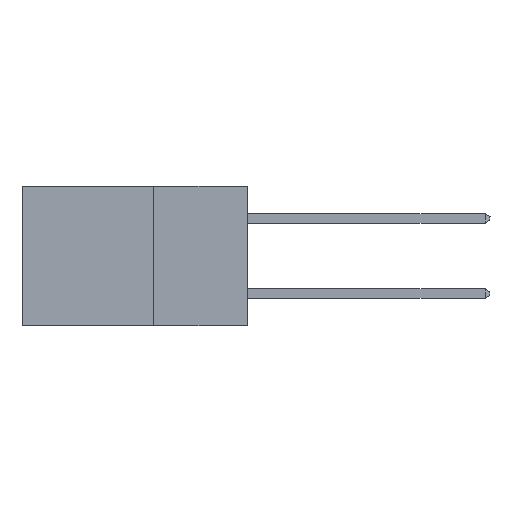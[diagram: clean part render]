
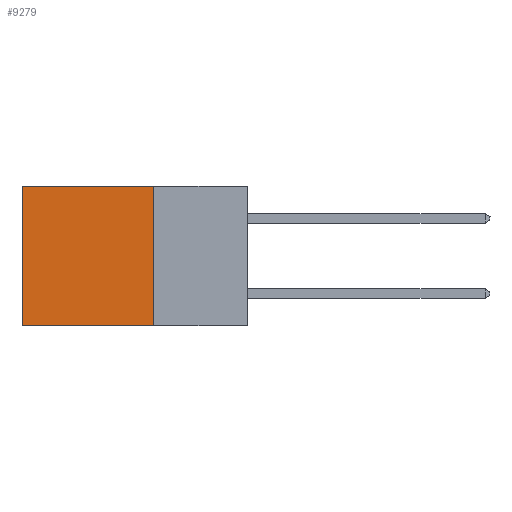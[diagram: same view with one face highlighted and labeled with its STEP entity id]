
A CAD part, left-side view. The second image highlights one B-rep face of the part: STEP entity #9279.
In plain terms, the highlighted planar face has unit normal (-1, 0, 0).
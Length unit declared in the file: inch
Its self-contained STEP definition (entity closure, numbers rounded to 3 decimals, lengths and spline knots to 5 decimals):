
#1099 = CARTESIAN_POINT ( 'NONE',  ( 0.2615, 0.6, -0.37 ) ) ;
#2013 = DIRECTION ( 'NONE',  ( 0., 1., 0. ) ) ;
#2723 = VECTOR ( 'NONE', #13078, 39.37008 ) ;
#2964 = VERTEX_POINT ( 'NONE', #15084 ) ;
#3114 = CARTESIAN_POINT ( 'NONE',  ( 0.2615, 0.25, -0.37 ) ) ;
#3133 = DIRECTION ( 'NONE',  ( 0., 0., -1. ) ) ;
#3724 = CARTESIAN_POINT ( 'NONE',  ( 0.2615, 0.6, 0. ) ) ;
#4052 = CARTESIAN_POINT ( 'NONE',  ( 0.2615, 0.25, -0.37 ) ) ;
#4297 = CARTESIAN_POINT ( 'NONE',  ( 0.2615, 0.6, -0.37 ) ) ;
#4444 = PLANE ( 'NONE',  #4728 ) ;
#4728 = AXIS2_PLACEMENT_3D ( 'NONE', #8635, #11301, #9491 ) ;
#5065 = ORIENTED_EDGE ( 'NONE', *, *, #6851, .T. ) ;
#5196 = EDGE_LOOP ( 'NONE', ( #5065, #15899, #11565, #14851 ) ) ;
#5509 = VECTOR ( 'NONE', #2013, 39.37008 ) ;
#6264 = EDGE_CURVE ( 'NONE', #2964, #8050, #11392, .T. ) ;
#6851 = EDGE_CURVE ( 'NONE', #14279, #11675, #14535, .T. ) ;
#7336 = EDGE_CURVE ( 'NONE', #2964, #14279, #8309, .T. ) ;
#7638 = CARTESIAN_POINT ( 'NONE',  ( 0.2615, 0.25, -0.37 ) ) ;
#8050 = VERTEX_POINT ( 'NONE', #4052 ) ;
#8309 = LINE ( 'NONE', #13406, #5509 ) ;
#8635 = CARTESIAN_POINT ( 'NONE',  ( 0.2615, 0.25, -0.37 ) ) ;
#9279 = ADVANCED_FACE ( 'NONE', ( #16297 ), #4444, .F. ) ;
#9491 = DIRECTION ( 'NONE',  ( 0., 0., -1. ) ) ;
#9801 = EDGE_CURVE ( 'NONE', #8050, #11675, #14704, .T. ) ;
#11045 = VECTOR ( 'NONE', #11546, 39.37008 ) ;
#11301 = DIRECTION ( 'NONE',  ( 1., 0., 0. ) ) ;
#11392 = LINE ( 'NONE', #7638, #11045 ) ;
#11546 = DIRECTION ( 'NONE',  ( 0., 0., -1. ) ) ;
#11565 = ORIENTED_EDGE ( 'NONE', *, *, #6264, .F. ) ;
#11675 = VERTEX_POINT ( 'NONE', #1099 ) ;
#13078 = DIRECTION ( 'NONE',  ( 0., 1., 0. ) ) ;
#13406 = CARTESIAN_POINT ( 'NONE',  ( 0.2615, 0.25, 0. ) ) ;
#14279 = VERTEX_POINT ( 'NONE', #3724 ) ;
#14535 = LINE ( 'NONE', #4297, #16119 ) ;
#14704 = LINE ( 'NONE', #3114, #2723 ) ;
#14851 = ORIENTED_EDGE ( 'NONE', *, *, #7336, .T. ) ;
#15084 = CARTESIAN_POINT ( 'NONE',  ( 0.2615, 0.25, 0. ) ) ;
#15899 = ORIENTED_EDGE ( 'NONE', *, *, #9801, .F. ) ;
#16119 = VECTOR ( 'NONE', #3133, 39.37008 ) ;
#16297 = FACE_OUTER_BOUND ( 'NONE', #5196, .T. ) ;
